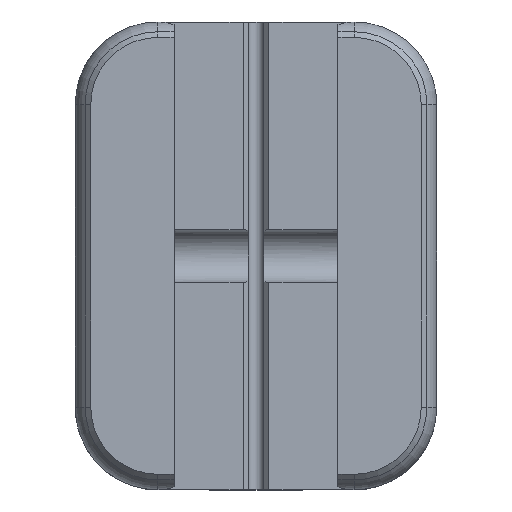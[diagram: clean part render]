
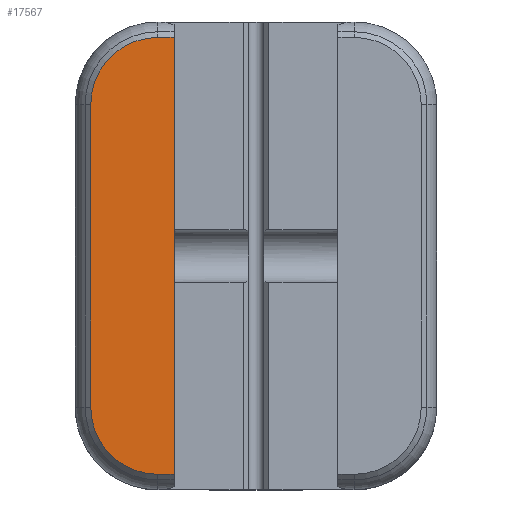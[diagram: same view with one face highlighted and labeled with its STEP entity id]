
A CAD part, top view. The second image highlights one B-rep face of the part: STEP entity #17567.
In plain terms, the highlighted planar face has unit normal (0, 0, 1).
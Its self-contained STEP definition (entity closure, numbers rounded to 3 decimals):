
#167=PLANE('',#19784);
#876=LINE('',#40964,#1623);
#879=LINE('',#40972,#1626);
#890=LINE('',#40999,#1637);
#893=LINE('',#41004,#1640);
#1623=VECTOR('',#24819,10.);
#1626=VECTOR('',#24828,10.);
#1637=VECTOR('',#24857,10.);
#1640=VECTOR('',#24864,10.);
#3492=FACE_OUTER_BOUND('',#4661,.T.);
#4661=EDGE_LOOP('',(#15877,#15878,#15879,#15880,#15881,#15882));
#6582=CIRCLE('',#19768,6.5);
#6583=CIRCLE('',#19771,6.5);
#8056=VERTEX_POINT('',#40956);
#8057=VERTEX_POINT('',#40958);
#8058=VERTEX_POINT('',#40962);
#8059=VERTEX_POINT('',#40966);
#8060=VERTEX_POINT('',#40970);
#8067=VERTEX_POINT('',#40998);
#10672=EDGE_CURVE('',#8056,#8057,#6582,.T.);
#10675=EDGE_CURVE('',#8058,#8056,#876,.T.);
#10677=EDGE_CURVE('',#8059,#8058,#6583,.T.);
#10679=EDGE_CURVE('',#8060,#8059,#879,.T.);
#10693=EDGE_CURVE('',#8057,#8067,#890,.T.);
#10696=EDGE_CURVE('',#8067,#8060,#893,.F.);
#15877=ORIENTED_EDGE('',*,*,#10693,.F.);
#15878=ORIENTED_EDGE('',*,*,#10672,.F.);
#15879=ORIENTED_EDGE('',*,*,#10675,.F.);
#15880=ORIENTED_EDGE('',*,*,#10677,.F.);
#15881=ORIENTED_EDGE('',*,*,#10679,.F.);
#15882=ORIENTED_EDGE('',*,*,#10696,.F.);
#17567=ADVANCED_FACE('',(#3492),#167,.F.);
#19768=AXIS2_PLACEMENT_3D('',#40959,#24813,#24814);
#19771=AXIS2_PLACEMENT_3D('',#40968,#24823,#24824);
#19784=AXIS2_PLACEMENT_3D('',#41006,#24866,#24867);
#24813=DIRECTION('center_axis',(0.,0.,
-1.));
#24814=DIRECTION('ref_axis',(-0.707,0.707,0.));
#24819=DIRECTION('',(0.,1.,0.));
#24823=DIRECTION('center_axis',(0.,0.,
-1.));
#24824=DIRECTION('ref_axis',(-0.707,-0.707,0.));
#24828=DIRECTION('',(-1.,0.,0.));
#24857=DIRECTION('',(1.,0.,0.));
#24864=DIRECTION('',(0.,1.,0.));
#24866=DIRECTION('center_axis',(0.,0.,
-1.));
#24867=DIRECTION('ref_axis',(1.,0.,0.));
#40956=CARTESIAN_POINT('',(-16.,69.653,-24.354));
#40958=CARTESIAN_POINT('',(-9.5,76.153,-24.354));
#40959=CARTESIAN_POINT('Origin',(-9.5,69.653,-24.354));
#40962=CARTESIAN_POINT('',(-16.,40.355,-24.354));
#40964=CARTESIAN_POINT('',(-16.,69.903,-24.354));
#40966=CARTESIAN_POINT('',(-9.5,33.855,-24.354));
#40968=CARTESIAN_POINT('Origin',(-9.5,40.355,-24.354));
#40970=CARTESIAN_POINT('',(-7.936,33.855,-24.354));
#40972=CARTESIAN_POINT('',(-10.135,33.855,-24.354));
#40998=CARTESIAN_POINT('',(-7.936,76.153,-24.354));
#40999=CARTESIAN_POINT('',(-10.135,76.153,-24.354));
#41004=CARTESIAN_POINT('',(-7.936,42.504,-24.354));
#41006=CARTESIAN_POINT('Origin',(-20.269,69.903,-24.354));
